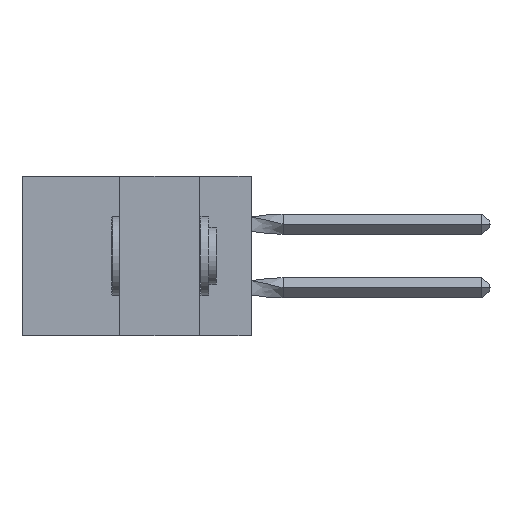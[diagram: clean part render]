
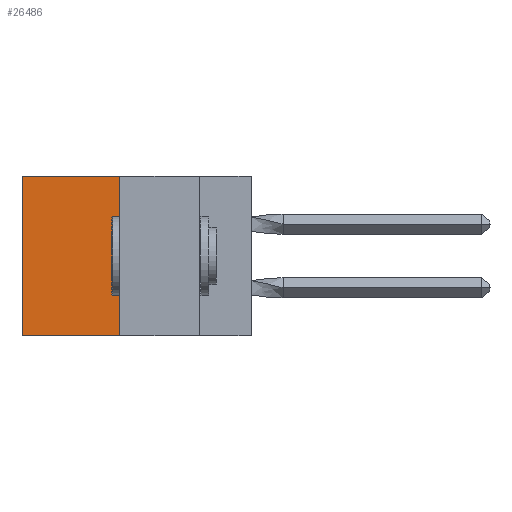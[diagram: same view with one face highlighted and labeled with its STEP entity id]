
A CAD part, left-side view. The second image highlights one B-rep face of the part: STEP entity #26486.
In plain terms, the highlighted planar face has unit normal (-1, 0, 0).
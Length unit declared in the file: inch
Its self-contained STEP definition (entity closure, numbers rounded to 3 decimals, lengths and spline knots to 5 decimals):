
#1101 = ORIENTED_EDGE ( 'NONE', *, *, #1325, .T. ) ;
#1141 = DIRECTION ( 'NONE',  ( 0., 1., 0. ) ) ;
#1162 = LINE ( 'NONE', #5782, #12080 ) ;
#1325 = EDGE_CURVE ( 'NONE', #9693, #19215, #20310, .T. ) ;
#1608 = DIRECTION ( 'NONE',  ( 0., 0., -1. ) ) ;
#2301 = DIRECTION ( 'NONE',  ( 0., 0., -1. ) ) ;
#4882 = FACE_OUTER_BOUND ( 'NONE', #5570, .T. ) ;
#5441 = VERTEX_POINT ( 'NONE', #25739 ) ;
#5570 = EDGE_LOOP ( 'NONE', ( #5688, #26476, #16989, #1101 ) ) ;
#5688 = ORIENTED_EDGE ( 'NONE', *, *, #17841, .T. ) ;
#5782 = CARTESIAN_POINT ( 'NONE',  ( 0.305, 0.72, -0.5 ) ) ;
#6693 = CARTESIAN_POINT ( 'NONE',  ( 0.305, 0.413, -0.5 ) ) ;
#7540 = VECTOR ( 'NONE', #19791, 39.37008 ) ;
#8956 = VECTOR ( 'NONE', #11200, 39.37008 ) ;
#9278 = CARTESIAN_POINT ( 'NONE',  ( 0.305, 0.413, -0.5 ) ) ;
#9486 = AXIS2_PLACEMENT_3D ( 'NONE', #10604, #10700, #2301 ) ;
#9693 = VERTEX_POINT ( 'NONE', #21850 ) ;
#10604 = CARTESIAN_POINT ( 'NONE',  ( 0.305, 0.413, -0.5 ) ) ;
#10700 = DIRECTION ( 'NONE',  ( 1., 0., 0. ) ) ;
#11200 = DIRECTION ( 'NONE',  ( 0., 1., 0. ) ) ;
#11823 = LINE ( 'NONE', #9278, #7540 ) ;
#12080 = VECTOR ( 'NONE', #1608, 39.37008 ) ;
#13706 = EDGE_CURVE ( 'NONE', #5441, #19601, #20506, .T. ) ;
#16117 = CARTESIAN_POINT ( 'NONE',  ( 0.305, 0.413, 0. ) ) ;
#16534 = EDGE_CURVE ( 'NONE', #9693, #5441, #11823, .T. ) ;
#16989 = ORIENTED_EDGE ( 'NONE', *, *, #16534, .F. ) ;
#17841 = EDGE_CURVE ( 'NONE', #19215, #19601, #1162, .T. ) ;
#18747 = CARTESIAN_POINT ( 'NONE',  ( 0.305, 0.72, 0. ) ) ;
#19215 = VERTEX_POINT ( 'NONE', #18747 ) ;
#19601 = VERTEX_POINT ( 'NONE', #24816 ) ;
#19791 = DIRECTION ( 'NONE',  ( 0., 0., -1. ) ) ;
#20310 = LINE ( 'NONE', #16117, #23954 ) ;
#20506 = LINE ( 'NONE', #6693, #8956 ) ;
#21850 = CARTESIAN_POINT ( 'NONE',  ( 0.305, 0.413, 0. ) ) ;
#23954 = VECTOR ( 'NONE', #1141, 39.37008 ) ;
#24816 = CARTESIAN_POINT ( 'NONE',  ( 0.305, 0.72, -0.5 ) ) ;
#24914 = PLANE ( 'NONE',  #9486 ) ;
#25739 = CARTESIAN_POINT ( 'NONE',  ( 0.305, 0.413, -0.5 ) ) ;
#26476 = ORIENTED_EDGE ( 'NONE', *, *, #13706, .F. ) ;
#26486 = ADVANCED_FACE ( 'NONE', ( #4882 ), #24914, .F. ) ;
